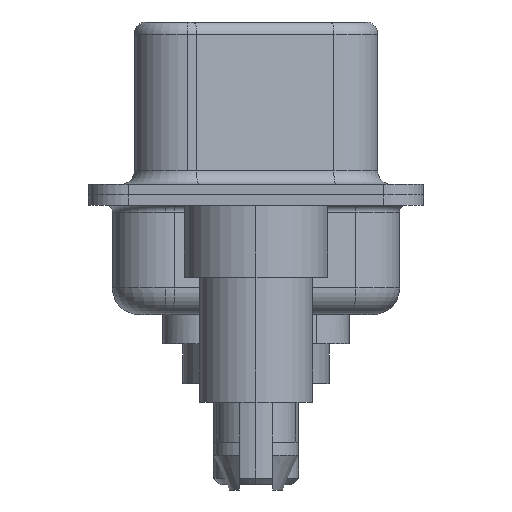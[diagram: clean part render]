
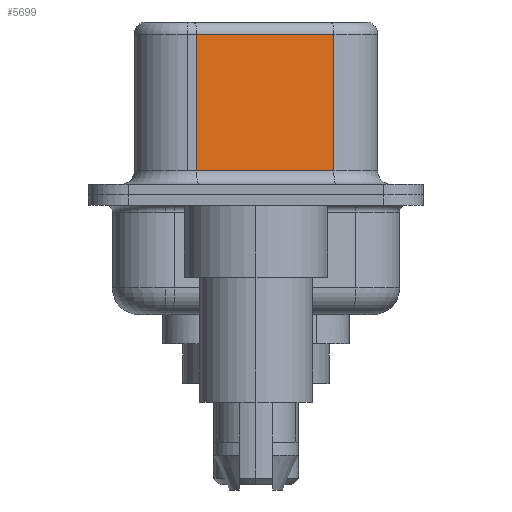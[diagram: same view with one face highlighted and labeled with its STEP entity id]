
A CAD part, left-side view. The second image highlights one B-rep face of the part: STEP entity #5699.
In plain terms, the highlighted planar face has unit normal (-0.985, -0.174, 0).
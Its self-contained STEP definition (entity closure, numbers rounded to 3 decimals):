
#9 = ORIENTED_EDGE ( 'NONE', *, *, #15834, .T. ) ;
#11 = EDGE_LOOP ( 'NONE', ( #3880, #12078, #11493, #9 ) ) ;
#235 = LINE ( 'NONE', #19108, #15703 ) ;
#1858 = CARTESIAN_POINT ( 'NONE',  ( 4.585, -2.927, 6.52 ) ) ;
#3374 = DIRECTION ( 'NONE',  ( 0.985, 0.174, 0. ) ) ;
#3558 = CARTESIAN_POINT ( 'NONE',  ( 4.585, -2.927, 6.02 ) ) ;
#3880 = ORIENTED_EDGE ( 'NONE', *, *, #12429, .F. ) ;
#4255 = VECTOR ( 'NONE', #9758, 1000. ) ;
#5699 = ADVANCED_FACE ( 'NONE', ( #6330 ), #10828, .F. ) ;
#5975 = VECTOR ( 'NONE', #12514, 1000. ) ;
#6271 = VERTEX_POINT ( 'NONE', #9043 ) ;
#6330 = FACE_OUTER_BOUND ( 'NONE', #11, .T. ) ;
#7919 = CARTESIAN_POINT ( 'NONE',  ( 4.585, -2.927, 6.52 ) ) ;
#8166 = EDGE_CURVE ( 'NONE', #9511, #18342, #235, .T. ) ;
#8627 = DIRECTION ( 'NONE',  ( 0., 0., -1. ) ) ;
#8827 = AXIS2_PLACEMENT_3D ( 'NONE', #1858, #3374, #13845 ) ;
#9043 = CARTESIAN_POINT ( 'NONE',  ( 4.585, -2.927, 6.02 ) ) ;
#9511 = VERTEX_POINT ( 'NONE', #13498 ) ;
#9758 = DIRECTION ( 'NONE',  ( 0.174, -0.985, 0. ) ) ;
#9777 = CARTESIAN_POINT ( 'NONE',  ( 3.675, 2.233, 0.9 ) ) ;
#10003 = VECTOR ( 'NONE', #15380, 1000. ) ;
#10828 = PLANE ( 'NONE',  #8827 ) ;
#11493 = ORIENTED_EDGE ( 'NONE', *, *, #8166, .T. ) ;
#12078 = ORIENTED_EDGE ( 'NONE', *, *, #13565, .T. ) ;
#12429 = EDGE_CURVE ( 'NONE', #6271, #14124, #17965, .T. ) ;
#12514 = DIRECTION ( 'NONE',  ( -0.174, 0.985, 0. ) ) ;
#13498 = CARTESIAN_POINT ( 'NONE',  ( 3.675, 2.233, 6.02 ) ) ;
#13565 = EDGE_CURVE ( 'NONE', #6271, #9511, #17931, .T. ) ;
#13845 = DIRECTION ( 'NONE',  ( -0.174, 0.985, 0. ) ) ;
#14124 = VERTEX_POINT ( 'NONE', #18400 ) ;
#15380 = DIRECTION ( 'NONE',  ( 0., 0., -1. ) ) ;
#15703 = VECTOR ( 'NONE', #8627, 1000. ) ;
#15834 = EDGE_CURVE ( 'NONE', #18342, #14124, #16192, .T. ) ;
#16192 = LINE ( 'NONE', #17219, #4255 ) ;
#17219 = CARTESIAN_POINT ( 'NONE',  ( 4.585, -2.927, 0.9 ) ) ;
#17931 = LINE ( 'NONE', #3558, #5975 ) ;
#17965 = LINE ( 'NONE', #7919, #10003 ) ;
#18342 = VERTEX_POINT ( 'NONE', #9777 ) ;
#18400 = CARTESIAN_POINT ( 'NONE',  ( 4.585, -2.927, 0.9 ) ) ;
#19108 = CARTESIAN_POINT ( 'NONE',  ( 3.675, 2.233, 6.52 ) ) ;
